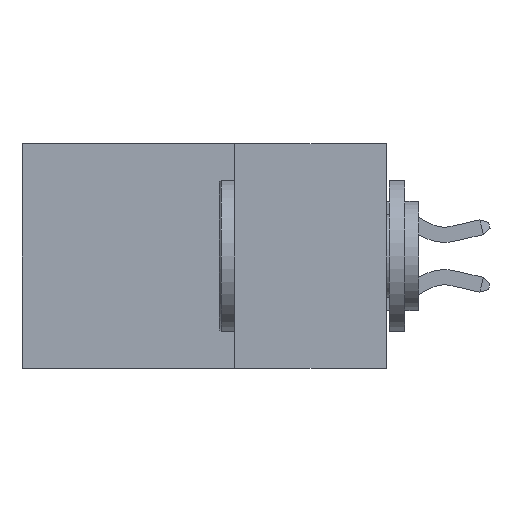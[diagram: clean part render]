
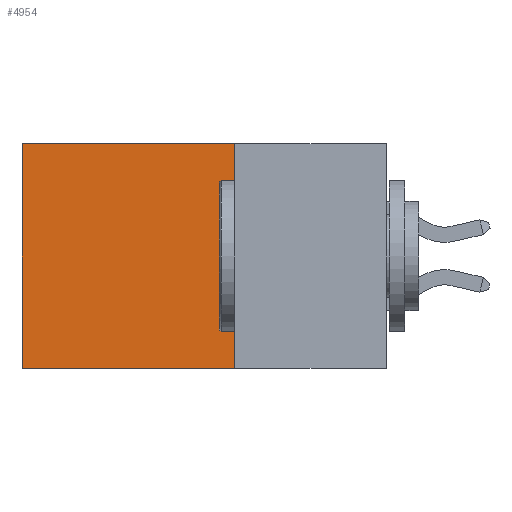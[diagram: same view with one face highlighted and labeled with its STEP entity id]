
A CAD part, left-side view. The second image highlights one B-rep face of the part: STEP entity #4954.
In plain terms, the highlighted planar face has unit normal (-1, 0, 0).
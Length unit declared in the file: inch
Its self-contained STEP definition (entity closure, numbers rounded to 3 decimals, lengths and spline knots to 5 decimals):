
#266 = EDGE_CURVE ( 'NONE', #3888, #19227, #6781, .T. ) ;
#589 = VECTOR ( 'NONE', #9245, 39.37008 ) ;
#1739 = EDGE_CURVE ( 'NONE', #3764, #19621, #12021, .T. ) ;
#3050 = CARTESIAN_POINT ( 'NONE',  ( 0.2615, 0.25, -0.37 ) ) ;
#3506 = CARTESIAN_POINT ( 'NONE',  ( 0.2615, 0.25, -0.37 ) ) ;
#3764 = VERTEX_POINT ( 'NONE', #13278 ) ;
#3888 = VERTEX_POINT ( 'NONE', #19407 ) ;
#4183 = CARTESIAN_POINT ( 'NONE',  ( 0.2615, 0.6, -0.37 ) ) ;
#4813 = VECTOR ( 'NONE', #16110, 39.37008 ) ;
#4897 = FACE_OUTER_BOUND ( 'NONE', #8817, .T. ) ;
#4954 = ADVANCED_FACE ( 'NONE', ( #4897 ), #15854, .F. ) ;
#5056 = LINE ( 'NONE', #3506, #16464 ) ;
#5848 = EDGE_CURVE ( 'NONE', #19621, #19227, #5056, .T. ) ;
#6422 = DIRECTION ( 'NONE',  ( 1., 0., 0. ) ) ;
#6781 = LINE ( 'NONE', #4183, #4813 ) ;
#7489 = LINE ( 'NONE', #10571, #19927 ) ;
#8310 = CARTESIAN_POINT ( 'NONE',  ( 0.2615, 0.6, -0.37 ) ) ;
#8727 = DIRECTION ( 'NONE',  ( 0., 1., 0. ) ) ;
#8817 = EDGE_LOOP ( 'NONE', ( #10999, #13373, #14602, #13280 ) ) ;
#9245 = DIRECTION ( 'NONE',  ( 0., 0., -1. ) ) ;
#9821 = CARTESIAN_POINT ( 'NONE',  ( 0.2615, 0.25, -0.37 ) ) ;
#10571 = CARTESIAN_POINT ( 'NONE',  ( 0.2615, 0.25, 0. ) ) ;
#10999 = ORIENTED_EDGE ( 'NONE', *, *, #266, .T. ) ;
#11614 = DIRECTION ( 'NONE',  ( 0., 1., 0. ) ) ;
#12021 = LINE ( 'NONE', #13729, #589 ) ;
#12390 = DIRECTION ( 'NONE',  ( 0., 0., -1. ) ) ;
#13278 = CARTESIAN_POINT ( 'NONE',  ( 0.2615, 0.25, 0. ) ) ;
#13280 = ORIENTED_EDGE ( 'NONE', *, *, #16147, .T. ) ;
#13373 = ORIENTED_EDGE ( 'NONE', *, *, #5848, .F. ) ;
#13729 = CARTESIAN_POINT ( 'NONE',  ( 0.2615, 0.25, -0.37 ) ) ;
#14602 = ORIENTED_EDGE ( 'NONE', *, *, #1739, .F. ) ;
#15854 = PLANE ( 'NONE',  #17401 ) ;
#16110 = DIRECTION ( 'NONE',  ( 0., 0., -1. ) ) ;
#16147 = EDGE_CURVE ( 'NONE', #3764, #3888, #7489, .T. ) ;
#16464 = VECTOR ( 'NONE', #11614, 39.37008 ) ;
#17401 = AXIS2_PLACEMENT_3D ( 'NONE', #3050, #6422, #12390 ) ;
#19227 = VERTEX_POINT ( 'NONE', #8310 ) ;
#19407 = CARTESIAN_POINT ( 'NONE',  ( 0.2615, 0.6, 0. ) ) ;
#19621 = VERTEX_POINT ( 'NONE', #9821 ) ;
#19927 = VECTOR ( 'NONE', #8727, 39.37008 ) ;
